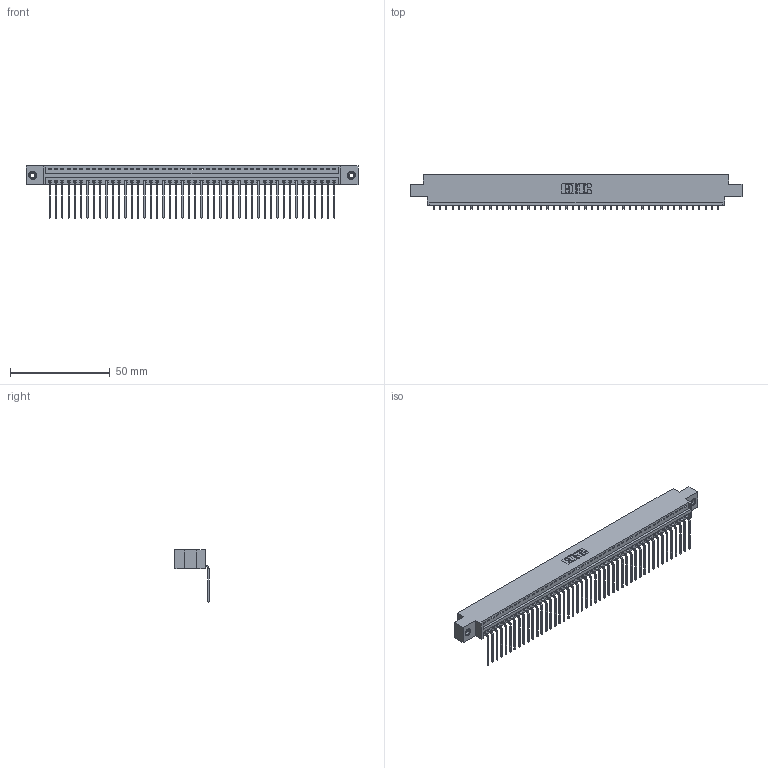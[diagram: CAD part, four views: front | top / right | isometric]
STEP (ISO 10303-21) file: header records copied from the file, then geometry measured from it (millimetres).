
FILE_DESCRIPTION (( 'STEP AP203' ), '1' );
FILE_NAME ('396-046-559-608.STEP', '2018-09-07T09:49:58', ( '' ), ( '' ), 'SwSTEP 2.0', 'SolidWorks 2016', '' );
FILE_SCHEMA (( 'CONFIG_CONTROL_DESIGN' ));
Length unit declared in the file: inch
Products named in the file (4): 346 Part_0.170 Offset - 0.156 Dia-TI; 345-292-001_558 559 Tail - 1; 345-250-001_345-250-003-102; 396-046-559-608
Assembly tree (49 placements, depth 2):
  396-046-559-608
    346 Part_0.170 Offset - 0.156 Dia-TI
    345-292-001_558 559 Tail - 1  x46
    345-250-001_345-250-003-102  x2
Bounding box: 166.62 x 17.08 x 26.16 mm (x, y, z)
Volume: 15969.3 mm3; surface area: 21099.2 mm2
Topology: 49 solids, 49 shells, 2946 faces, 8849 edges, 5830 vertices
Faces by surface type: plane 2044, cylinder 886, cone 12, torus 4
Entity records: 29412 total; most frequent: CARTESIAN_POINT 5025, ORIENTED_EDGE 4998, DIRECTION 4453, EDGE_CURVE 2499, LINE 2163, VECTOR 2163, VERTEX_POINT 1660, AXIS2_PLACEMENT_3D 1145
